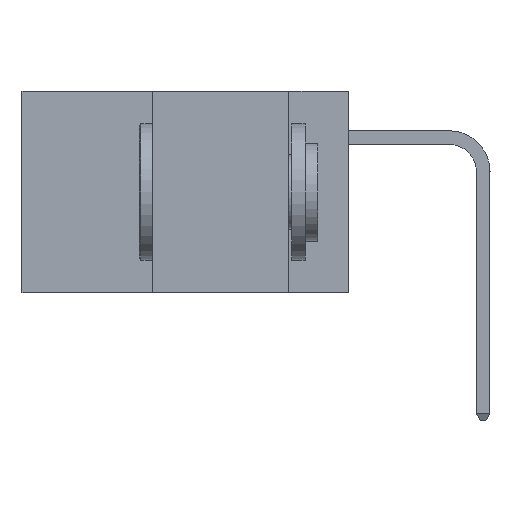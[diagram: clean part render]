
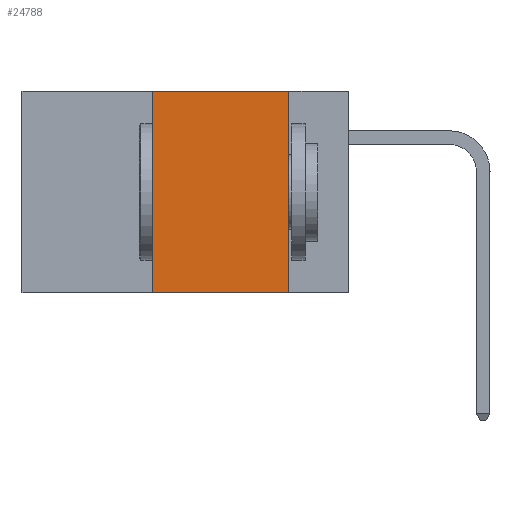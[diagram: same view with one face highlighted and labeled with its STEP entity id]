
A CAD part, left-side view. The second image highlights one B-rep face of the part: STEP entity #24788.
In plain terms, the highlighted planar face has unit normal (-1, 0, 0).
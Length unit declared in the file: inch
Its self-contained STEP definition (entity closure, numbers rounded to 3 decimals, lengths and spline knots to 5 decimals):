
#1015 = EDGE_CURVE ( 'NONE', #14864, #27115, #31985, .T. ) ;
#4762 = ORIENTED_EDGE ( 'NONE', *, *, #16736, .T. ) ;
#5427 = VECTOR ( 'NONE', #11575, 39.37008 ) ;
#5804 = CARTESIAN_POINT ( 'NONE',  ( 0., 0.36, -0.37 ) ) ;
#6804 = PLANE ( 'NONE',  #7772 ) ;
#7772 = AXIS2_PLACEMENT_3D ( 'NONE', #19423, #29057, #10001 ) ;
#7972 = EDGE_CURVE ( 'NONE', #27115, #17637, #11553, .T. ) ;
#8252 = ORIENTED_EDGE ( 'NONE', *, *, #7972, .F. ) ;
#10001 = DIRECTION ( 'NONE',  ( 0., 0., -1. ) ) ;
#11553 = LINE ( 'NONE', #19210, #27494 ) ;
#11566 = CARTESIAN_POINT ( 'NONE',  ( 0., 0.36, 0. ) ) ;
#11575 = DIRECTION ( 'NONE',  ( 0., -1., 0. ) ) ;
#13849 = LINE ( 'NONE', #27447, #5427 ) ;
#14864 = VERTEX_POINT ( 'NONE', #11566 ) ;
#15145 = ORIENTED_EDGE ( 'NONE', *, *, #37240, .F. ) ;
#15466 = CARTESIAN_POINT ( 'NONE',  ( 0., 0.36, 0. ) ) ;
#16123 = DIRECTION ( 'NONE',  ( 0., 0., -1. ) ) ;
#16736 = EDGE_CURVE ( 'NONE', #30820, #17637, #13849, .T. ) ;
#17021 = VECTOR ( 'NONE', #35011, 39.37008 ) ;
#17637 = VERTEX_POINT ( 'NONE', #18382 ) ;
#18382 = CARTESIAN_POINT ( 'NONE',  ( 0., 0.11, -0.37 ) ) ;
#19210 = CARTESIAN_POINT ( 'NONE',  ( 0., 0.11, 0. ) ) ;
#19423 = CARTESIAN_POINT ( 'NONE',  ( 0., 0.6, 0. ) ) ;
#22746 = CARTESIAN_POINT ( 'NONE',  ( 0., 0.11, 0. ) ) ;
#24788 = ADVANCED_FACE ( 'NONE', ( #28091 ), #6804, .F. ) ;
#27115 = VERTEX_POINT ( 'NONE', #22746 ) ;
#27447 = CARTESIAN_POINT ( 'NONE',  ( 0., 0.6, -0.37 ) ) ;
#27494 = VECTOR ( 'NONE', #16123, 39.37008 ) ;
#28091 = FACE_OUTER_BOUND ( 'NONE', #29159, .T. ) ;
#29057 = DIRECTION ( 'NONE',  ( 1., 0., 0. ) ) ;
#29159 = EDGE_LOOP ( 'NONE', ( #8252, #39033, #15145, #4762 ) ) ;
#30157 = VECTOR ( 'NONE', #34554, 39.37008 ) ;
#30820 = VERTEX_POINT ( 'NONE', #5804 ) ;
#31837 = CARTESIAN_POINT ( 'NONE',  ( 0., 0.6, 0. ) ) ;
#31985 = LINE ( 'NONE', #31837, #17021 ) ;
#34554 = DIRECTION ( 'NONE',  ( 0., 0., 1. ) ) ;
#35011 = DIRECTION ( 'NONE',  ( 0., -1., 0. ) ) ;
#37240 = EDGE_CURVE ( 'NONE', #30820, #14864, #38552, .T. ) ;
#38552 = LINE ( 'NONE', #15466, #30157 ) ;
#39033 = ORIENTED_EDGE ( 'NONE', *, *, #1015, .F. ) ;
